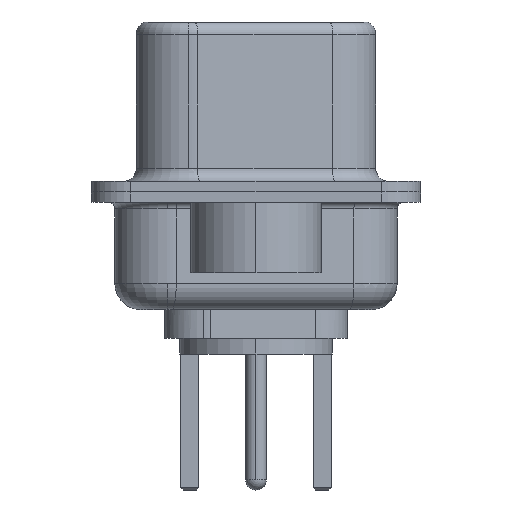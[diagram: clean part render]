
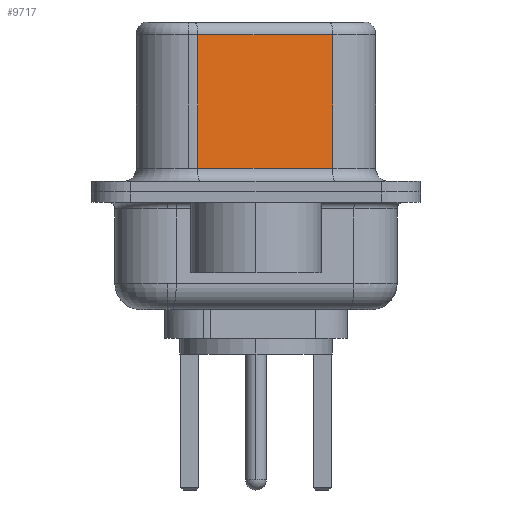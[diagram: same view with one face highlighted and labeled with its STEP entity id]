
A CAD part, left-side view. The second image highlights one B-rep face of the part: STEP entity #9717.
In plain terms, the highlighted planar face has unit normal (-0.985, -0.174, 0).
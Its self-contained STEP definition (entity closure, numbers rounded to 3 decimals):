
#340 = EDGE_CURVE ( 'NONE', #12852, #3041, #16198, .T. ) ;
#613 = ORIENTED_EDGE ( 'NONE', *, *, #19056, .T. ) ;
#695 = EDGE_CURVE ( 'NONE', #12852, #14533, #10507, .T. ) ;
#854 = DIRECTION ( 'NONE',  ( 0.985, 0.174, 0. ) ) ;
#1236 = ORIENTED_EDGE ( 'NONE', *, *, #340, .F. ) ;
#1336 = ORIENTED_EDGE ( 'NONE', *, *, #695, .T. ) ;
#2048 = VERTEX_POINT ( 'NONE', #11801 ) ;
#2178 = ORIENTED_EDGE ( 'NONE', *, *, #14072, .T. ) ;
#2201 = CARTESIAN_POINT ( 'NONE',  ( 4.585, -2.927, 0.9 ) ) ;
#2353 = PLANE ( 'NONE',  #12002 ) ;
#3041 = VERTEX_POINT ( 'NONE', #19023 ) ;
#3856 = LINE ( 'NONE', #10097, #19507 ) ;
#4855 = VECTOR ( 'NONE', #8228, 1000. ) ;
#5627 = DIRECTION ( 'NONE',  ( 0., 0., -1. ) ) ;
#6331 = DIRECTION ( 'NONE',  ( -0.174, 0.985, 0. ) ) ;
#8228 = DIRECTION ( 'NONE',  ( 0.174, -0.985, 0. ) ) ;
#9626 = DIRECTION ( 'NONE',  ( 0., 0., -1. ) ) ;
#9717 = ADVANCED_FACE ( 'NONE', ( #14422 ), #2353, .F. ) ;
#9936 = CARTESIAN_POINT ( 'NONE',  ( 4.585, -2.927, 6.52 ) ) ;
#10024 = VECTOR ( 'NONE', #6331, 1000. ) ;
#10097 = CARTESIAN_POINT ( 'NONE',  ( 3.675, 2.233, 6.52 ) ) ;
#10507 = LINE ( 'NONE', #11223, #10024 ) ;
#10802 = CARTESIAN_POINT ( 'NONE',  ( 4.585, -2.927, 6.02 ) ) ;
#11222 = VECTOR ( 'NONE', #9626, 1000. ) ;
#11223 = CARTESIAN_POINT ( 'NONE',  ( 4.585, -2.927, 6.02 ) ) ;
#11481 = DIRECTION ( 'NONE',  ( -0.174, 0.985, 0. ) ) ;
#11801 = CARTESIAN_POINT ( 'NONE',  ( 3.675, 2.233, 0.9 ) ) ;
#12002 = AXIS2_PLACEMENT_3D ( 'NONE', #9936, #854, #11481 ) ;
#12426 = CARTESIAN_POINT ( 'NONE',  ( 4.585, -2.927, 6.52 ) ) ;
#12852 = VERTEX_POINT ( 'NONE', #10802 ) ;
#13780 = EDGE_LOOP ( 'NONE', ( #1236, #1336, #613, #2178 ) ) ;
#14072 = EDGE_CURVE ( 'NONE', #2048, #3041, #16911, .T. ) ;
#14422 = FACE_OUTER_BOUND ( 'NONE', #13780, .T. ) ;
#14533 = VERTEX_POINT ( 'NONE', #14893 ) ;
#14893 = CARTESIAN_POINT ( 'NONE',  ( 3.675, 2.233, 6.02 ) ) ;
#16198 = LINE ( 'NONE', #12426, #11222 ) ;
#16911 = LINE ( 'NONE', #2201, #4855 ) ;
#19023 = CARTESIAN_POINT ( 'NONE',  ( 4.585, -2.927, 0.9 ) ) ;
#19056 = EDGE_CURVE ( 'NONE', #14533, #2048, #3856, .T. ) ;
#19507 = VECTOR ( 'NONE', #5627, 1000. ) ;
